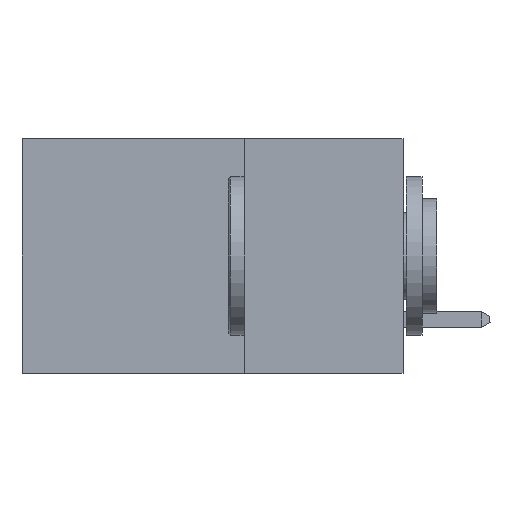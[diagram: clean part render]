
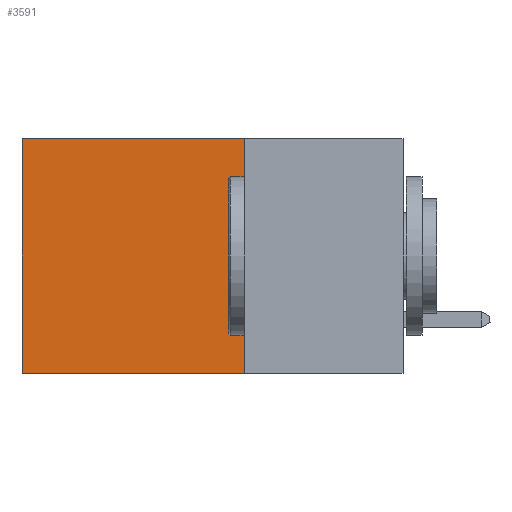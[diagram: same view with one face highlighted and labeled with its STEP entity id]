
A CAD part, left-side view. The second image highlights one B-rep face of the part: STEP entity #3591.
In plain terms, the highlighted planar face has unit normal (-1, 0, 0).
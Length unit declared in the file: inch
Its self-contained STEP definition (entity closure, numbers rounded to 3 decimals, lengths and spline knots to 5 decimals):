
#292 = DIRECTION ( 'NONE',  ( 0., 0., -1. ) ) ;
#344 = ORIENTED_EDGE ( 'NONE', *, *, #699, .T. ) ;
#699 = EDGE_CURVE ( 'NONE', #1925, #8164, #13173, .T. ) ;
#1494 = CARTESIAN_POINT ( 'NONE',  ( 0.2875, 0.6, 0. ) ) ;
#1760 = LINE ( 'NONE', #7889, #6282 ) ;
#1925 = VERTEX_POINT ( 'NONE', #1494 ) ;
#3315 = VERTEX_POINT ( 'NONE', #10654 ) ;
#3591 = ADVANCED_FACE ( 'NONE', ( #9984 ), #5294, .F. ) ;
#4351 = DIRECTION ( 'NONE',  ( 0., 1., 0. ) ) ;
#4813 = ORIENTED_EDGE ( 'NONE', *, *, #10689, .T. ) ;
#5294 = PLANE ( 'NONE',  #11716 ) ;
#5339 = DIRECTION ( 'NONE',  ( 0., 1., 0. ) ) ;
#5962 = VECTOR ( 'NONE', #12838, 39.37008 ) ;
#6015 = VERTEX_POINT ( 'NONE', #8377 ) ;
#6282 = VECTOR ( 'NONE', #4351, 39.37008 ) ;
#6487 = ORIENTED_EDGE ( 'NONE', *, *, #14108, .F. ) ;
#6524 = CARTESIAN_POINT ( 'NONE',  ( 0.2875, 0.6, 0. ) ) ;
#6600 = CARTESIAN_POINT ( 'NONE',  ( 0.2875, 0.25, 0. ) ) ;
#7889 = CARTESIAN_POINT ( 'NONE',  ( 0.2875, 0.25, -0.37 ) ) ;
#8115 = VECTOR ( 'NONE', #5339, 39.37008 ) ;
#8164 = VERTEX_POINT ( 'NONE', #15567 ) ;
#8268 = CARTESIAN_POINT ( 'NONE',  ( 0.2875, 0.25, 0. ) ) ;
#8377 = CARTESIAN_POINT ( 'NONE',  ( 0.2875, 0.25, 0. ) ) ;
#8906 = LINE ( 'NONE', #9934, #8115 ) ;
#9658 = DIRECTION ( 'NONE',  ( 0., 0., -1. ) ) ;
#9934 = CARTESIAN_POINT ( 'NONE',  ( 0.2875, 0.25, 0. ) ) ;
#9984 = FACE_OUTER_BOUND ( 'NONE', #10415, .T. ) ;
#10415 = EDGE_LOOP ( 'NONE', ( #344, #6487, #12684, #4813 ) ) ;
#10654 = CARTESIAN_POINT ( 'NONE',  ( 0.2875, 0.25, -0.37 ) ) ;
#10689 = EDGE_CURVE ( 'NONE', #6015, #1925, #8906, .T. ) ;
#11593 = VECTOR ( 'NONE', #9658, 39.37008 ) ;
#11716 = AXIS2_PLACEMENT_3D ( 'NONE', #6600, #15292, #292 ) ;
#12684 = ORIENTED_EDGE ( 'NONE', *, *, #16074, .F. ) ;
#12838 = DIRECTION ( 'NONE',  ( 0., 0., -1. ) ) ;
#13173 = LINE ( 'NONE', #6524, #5962 ) ;
#14108 = EDGE_CURVE ( 'NONE', #3315, #8164, #1760, .T. ) ;
#14522 = LINE ( 'NONE', #8268, #11593 ) ;
#15292 = DIRECTION ( 'NONE',  ( 1., 0., 0. ) ) ;
#15567 = CARTESIAN_POINT ( 'NONE',  ( 0.2875, 0.6, -0.37 ) ) ;
#16074 = EDGE_CURVE ( 'NONE', #6015, #3315, #14522, .T. ) ;
